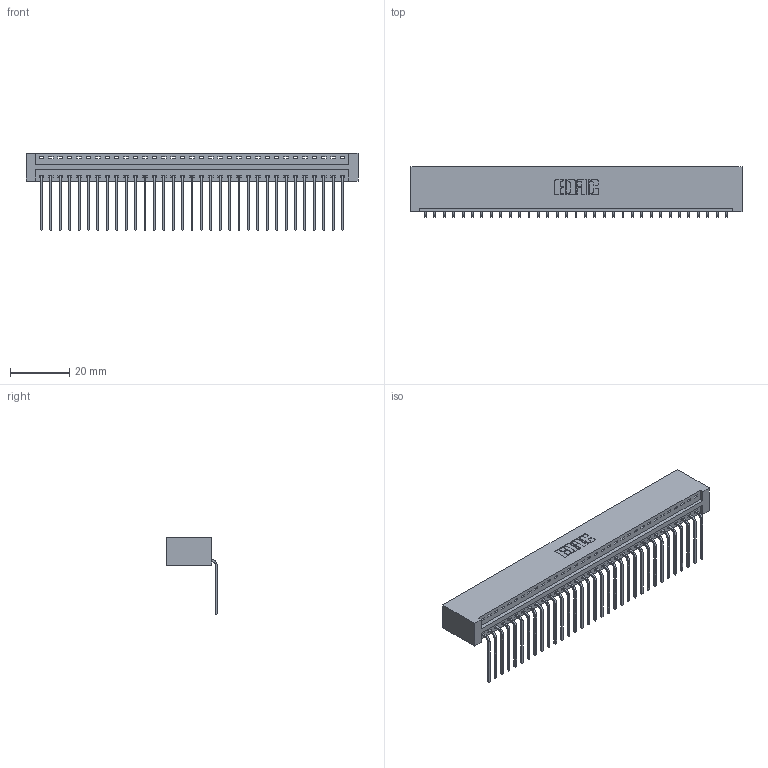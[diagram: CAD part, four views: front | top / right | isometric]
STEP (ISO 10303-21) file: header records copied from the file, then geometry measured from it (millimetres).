
FILE_DESCRIPTION (( 'STEP AP203' ), '1' );
FILE_NAME ('396-033-559-101.STEP', '2019-10-31T22:03:16', ( '' ), ( '' ), 'SwSTEP 2.0', 'SolidWorks 2016', '' );
FILE_SCHEMA (( 'CONFIG_CONTROL_DESIGN' ));
Length unit declared in the file: inch
Products named in the file (3): 346 Part_No Mounting Lugs; 345-292-001_558 559 Tail - 1; 396-033-559-101
Assembly tree (34 placements, depth 2):
  396-033-559-101
    346 Part_No Mounting Lugs
    345-292-001_558 559 Tail - 1  x33
Bounding box: 112.01 x 17.08 x 26.16 mm (x, y, z)
Volume: 11319.6 mm3; surface area: 14781.9 mm2
Topology: 34 solids, 34 shells, 2094 faces, 6311 edges, 4162 vertices
Faces by surface type: plane 1458, cylinder 636
Entity records: 21499 total; most frequent: CARTESIAN_POINT 3695, ORIENTED_EDGE 3662, DIRECTION 3265, EDGE_CURVE 1831, LINE 1575, VECTOR 1575, VERTEX_POINT 1218, AXIS2_PLACEMENT_3D 845
